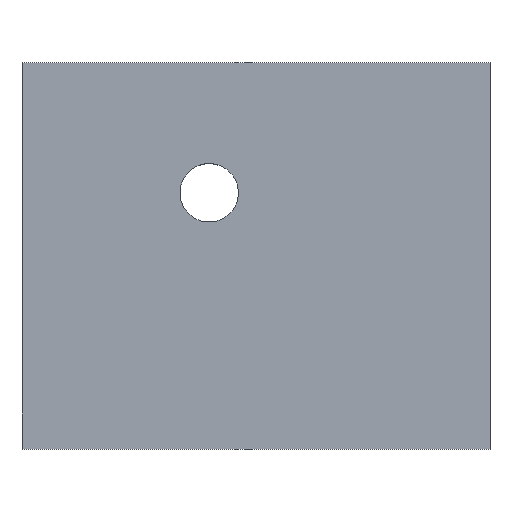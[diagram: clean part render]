
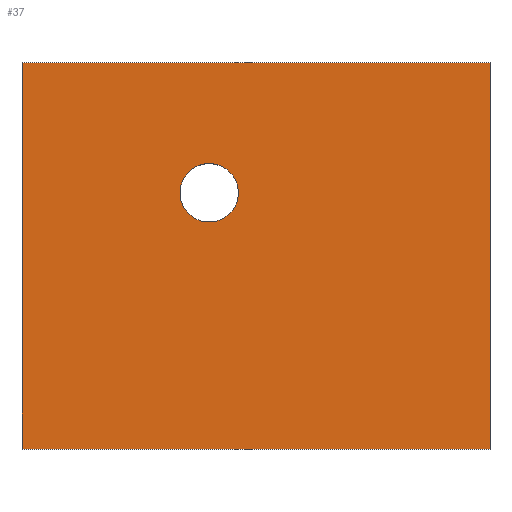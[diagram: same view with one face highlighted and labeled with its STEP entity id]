
A CAD part, top view. The second image highlights one B-rep face of the part: STEP entity #37.
In plain terms, the highlighted planar face has unit normal (0, 0, 1).
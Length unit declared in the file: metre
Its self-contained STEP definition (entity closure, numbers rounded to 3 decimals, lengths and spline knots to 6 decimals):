
#37=ADVANCED_FACE('0:4716',(#73,#74),#75,.F.);
#73=FACE_OUTER_BOUND('',#107,.T.);
#74=FACE_BOUND('',#108,.T.);
#75=PLANE('',#109);
#107=EDGE_LOOP('',(#145,#146,#147,#148));
#108=EDGE_LOOP('',(#149,#150));
#109=AXIS2_PLACEMENT_3D('',#151,#152,#153);
#145=ORIENTED_EDGE('',*,*,#206,.T.);
#146=ORIENTED_EDGE('',*,*,#207,.T.);
#147=ORIENTED_EDGE('',*,*,#208,.T.);
#148=ORIENTED_EDGE('',*,*,#209,.T.);
#149=ORIENTED_EDGE('',*,*,#201,.F.);
#150=ORIENTED_EDGE('',*,*,#203,.F.);
#151=CARTESIAN_POINT('',(-0.007485,0.055507,0.195006));
#152=DIRECTION('',(0.0,0.0,-1.0));
#153=DIRECTION('',(0.0,-1.0,0.0));
#201=EDGE_CURVE('0:4746',#230,#226,#232,.F.);
#203=EDGE_CURVE('0:4746',#226,#230,#234,.F.);
#206=EDGE_CURVE('0:4749',#237,#238,#239,.F.);
#207=EDGE_CURVE('0:4752',#238,#240,#241,.F.);
#208=EDGE_CURVE('0:4755',#240,#242,#243,.F.);
#209=EDGE_CURVE('0:4758',#242,#237,#244,.F.);
#226=VERTEX_POINT('',#265);
#230=VERTEX_POINT('',#270);
#232=CIRCLE('',#273,0.00125);
#234=CIRCLE('',#275,0.00125);
#237=VERTEX_POINT('',#278);
#238=VERTEX_POINT('',#279);
#239=LINE('',#280,#281);
#240=VERTEX_POINT('',#282);
#241=LINE('',#283,#284);
#242=VERTEX_POINT('',#285);
#243=LINE('',#286,#287);
#244=LINE('',#288,#289);
#265=CARTESIAN_POINT('',(-0.006601,0.047841,0.195006));
#270=CARTESIAN_POINT('',(-0.008369,0.046073,0.195006));
#273=AXIS2_PLACEMENT_3D('',#321,#322,#323);
#275=AXIS2_PLACEMENT_3D('',#324,#325,#326);
#278=CARTESIAN_POINT('',(0.004515,0.052507,0.195006));
#279=CARTESIAN_POINT('',(-0.015485,0.052507,0.195006));
#280=CARTESIAN_POINT('',(-0.006485,0.052507,0.195006));
#281=VECTOR('',#330,1.0);
#282=CARTESIAN_POINT('',(-0.015485,0.036007,0.195006));
#283=CARTESIAN_POINT('',(-0.015485,0.049882,0.195006));
#284=VECTOR('',#331,1.0);
#285=CARTESIAN_POINT('',(0.004515,0.036007,0.195006));
#286=CARTESIAN_POINT('',(-0.006485,0.036007,0.195006));
#287=VECTOR('',#332,1.0);
#288=CARTESIAN_POINT('',(0.004515,0.049882,0.195006));
#289=VECTOR('',#333,1.0);
#321=CARTESIAN_POINT('',(-0.007485,0.046957,0.195006));
#322=DIRECTION('',(0.0,0.0,-1.0));
#323=DIRECTION('',(0.707,0.707,0.0));
#324=CARTESIAN_POINT('',(-0.007485,0.046957,0.195006));
#325=DIRECTION('',(0.0,0.0,-1.0));
#326=DIRECTION('',(0.707,0.707,0.0));
#330=DIRECTION('',(1.0,0.0,0.0));
#331=DIRECTION('',(0.0,1.0,0.0));
#332=DIRECTION('',(-1.0,0.0,0.0));
#333=DIRECTION('',(0.0,-1.0,0.0));
